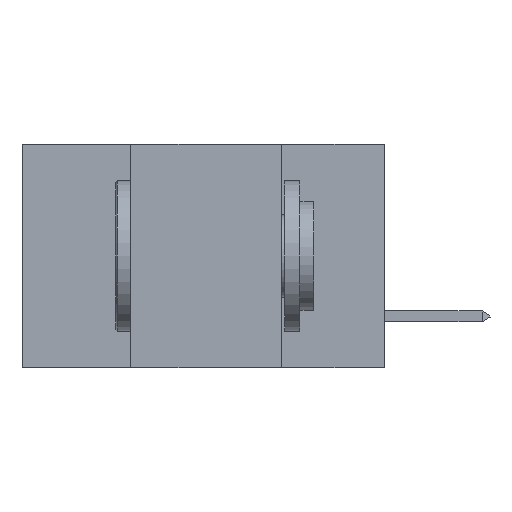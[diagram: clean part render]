
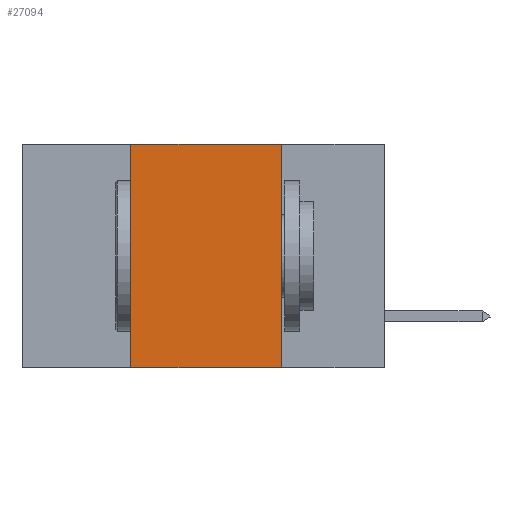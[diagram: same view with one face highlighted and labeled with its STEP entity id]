
A CAD part, left-side view. The second image highlights one B-rep face of the part: STEP entity #27094.
In plain terms, the highlighted planar face has unit normal (-1, 0, 0).
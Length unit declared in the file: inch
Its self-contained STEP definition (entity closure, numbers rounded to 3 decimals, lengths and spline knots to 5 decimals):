
#470 = VECTOR ( 'NONE', #8504, 39.37008 ) ;
#1086 = VERTEX_POINT ( 'NONE', #8715 ) ;
#1304 = DIRECTION ( 'NONE',  ( 1., 0., 0. ) ) ;
#2803 = CARTESIAN_POINT ( 'NONE',  ( 0., 0.42, 0. ) ) ;
#6288 = CARTESIAN_POINT ( 'NONE',  ( 0., 0.6, -0.37 ) ) ;
#6425 = ORIENTED_EDGE ( 'NONE', *, *, #27338, .F. ) ;
#6533 = CARTESIAN_POINT ( 'NONE',  ( 0., 0.17, 0. ) ) ;
#7200 = ORIENTED_EDGE ( 'NONE', *, *, #18727, .T. ) ;
#8504 = DIRECTION ( 'NONE',  ( 0., 0., -1. ) ) ;
#8507 = EDGE_CURVE ( 'NONE', #25121, #1086, #23693, .T. ) ;
#8715 = CARTESIAN_POINT ( 'NONE',  ( 0., 0.17, 0. ) ) ;
#9539 = DIRECTION ( 'NONE',  ( 0., 0., 1. ) ) ;
#10920 = CARTESIAN_POINT ( 'NONE',  ( 0., 0.42, -0.37 ) ) ;
#11321 = CARTESIAN_POINT ( 'NONE',  ( 0., 0.42, 0. ) ) ;
#11974 = DIRECTION ( 'NONE',  ( 0., 0., -1. ) ) ;
#12746 = ORIENTED_EDGE ( 'NONE', *, *, #13903, .F. ) ;
#13903 = EDGE_CURVE ( 'NONE', #14743, #25121, #24485, .T. ) ;
#14299 = ORIENTED_EDGE ( 'NONE', *, *, #8507, .F. ) ;
#14518 = CARTESIAN_POINT ( 'NONE',  ( 0., 0.17, -0.37 ) ) ;
#14743 = VERTEX_POINT ( 'NONE', #10920 ) ;
#17679 = VECTOR ( 'NONE', #27549, 39.37008 ) ;
#17715 = DIRECTION ( 'NONE',  ( 0., -1., 0. ) ) ;
#18213 = PLANE ( 'NONE',  #24527 ) ;
#18303 = CARTESIAN_POINT ( 'NONE',  ( 0., 0.6, 0. ) ) ;
#18438 = LINE ( 'NONE', #6533, #470 ) ;
#18727 = EDGE_CURVE ( 'NONE', #14743, #22682, #19687, .T. ) ;
#19345 = EDGE_LOOP ( 'NONE', ( #6425, #14299, #12746, #7200 ) ) ;
#19687 = LINE ( 'NONE', #6288, #17679 ) ;
#20357 = VECTOR ( 'NONE', #17715, 39.37008 ) ;
#22682 = VERTEX_POINT ( 'NONE', #14518 ) ;
#23693 = LINE ( 'NONE', #26199, #20357 ) ;
#24136 = FACE_OUTER_BOUND ( 'NONE', #19345, .T. ) ;
#24147 = VECTOR ( 'NONE', #9539, 39.37008 ) ;
#24485 = LINE ( 'NONE', #11321, #24147 ) ;
#24527 = AXIS2_PLACEMENT_3D ( 'NONE', #18303, #1304, #11974 ) ;
#25121 = VERTEX_POINT ( 'NONE', #2803 ) ;
#26199 = CARTESIAN_POINT ( 'NONE',  ( 0., 0.6, 0. ) ) ;
#27094 = ADVANCED_FACE ( 'NONE', ( #24136 ), #18213, .F. ) ;
#27338 = EDGE_CURVE ( 'NONE', #1086, #22682, #18438, .T. ) ;
#27549 = DIRECTION ( 'NONE',  ( 0., -1., 0. ) ) ;
